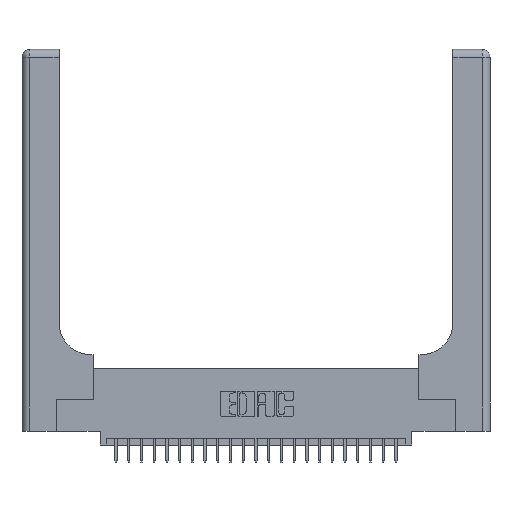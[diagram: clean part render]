
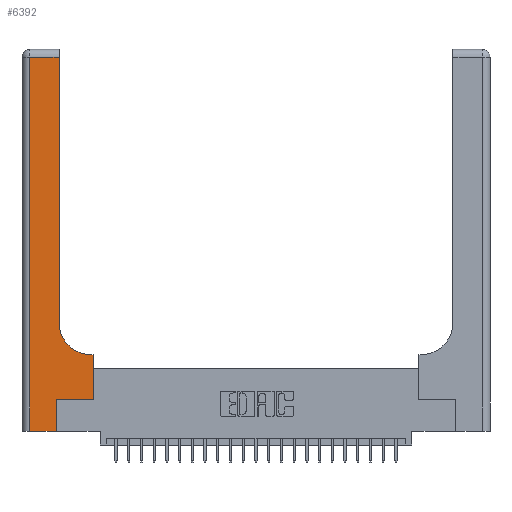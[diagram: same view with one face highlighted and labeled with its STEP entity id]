
A CAD part, top view. The second image highlights one B-rep face of the part: STEP entity #6392.
In plain terms, the highlighted planar face has unit normal (0, 0, 1).
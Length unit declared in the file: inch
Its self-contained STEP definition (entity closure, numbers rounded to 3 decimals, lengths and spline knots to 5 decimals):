
#55 = CARTESIAN_POINT ( 'NONE',  ( 0.5585, 0.25, 0.37 ) ) ;
#533 = VERTEX_POINT ( 'NONE', #17610 ) ;
#678 = CARTESIAN_POINT ( 'NONE',  ( 0.5585, 0.25, 0.37 ) ) ;
#694 = ORIENTED_EDGE ( 'NONE', *, *, #7546, .T. ) ;
#729 = LINE ( 'NONE', #22883, #1784 ) ;
#763 = DIRECTION ( 'NONE',  ( 1., 0., 0. ) ) ;
#1290 = CARTESIAN_POINT ( 'NONE',  ( 0.269, 0., 0.37 ) ) ;
#1412 = CARTESIAN_POINT ( 'NONE',  ( 0.2915, 0.85, 0.37 ) ) ;
#1784 = VECTOR ( 'NONE', #10490, 39.37008 ) ;
#1801 = DIRECTION ( 'NONE',  ( -1., 0., 0. ) ) ;
#2738 = DIRECTION ( 'NONE',  ( 0., -1., 0. ) ) ;
#2755 = ORIENTED_EDGE ( 'NONE', *, *, #14504, .T. ) ;
#3566 = CARTESIAN_POINT ( 'NONE',  ( 0.5415, 0.6, 0.37 ) ) ;
#4419 = LINE ( 'NONE', #8686, #8423 ) ;
#4421 = CARTESIAN_POINT ( 'NONE',  ( 0.269, 0.25, 0.37 ) ) ;
#4665 = LINE ( 'NONE', #6652, #6170 ) ;
#5395 = ORIENTED_EDGE ( 'NONE', *, *, #18539, .T. ) ;
#6170 = VECTOR ( 'NONE', #24715, 39.37008 ) ;
#6392 = ADVANCED_FACE ( 'NONE', ( #23810 ), #13932, .F. ) ;
#6423 = LINE ( 'NONE', #4421, #9833 ) ;
#6580 = ORIENTED_EDGE ( 'NONE', *, *, #19570, .T. ) ;
#6650 = LINE ( 'NONE', #9058, #25656 ) ;
#6652 = CARTESIAN_POINT ( 'NONE',  ( 0., 2.94, 0.37 ) ) ;
#6857 = VERTEX_POINT ( 'NONE', #10459 ) ;
#6976 = DIRECTION ( 'NONE',  ( 0., 1., 0. ) ) ;
#7003 = EDGE_LOOP ( 'NONE', ( #19323, #19224, #11215, #21803, #2755, #6580, #694, #5395, #24753 ) ) ;
#7546 = EDGE_CURVE ( 'NONE', #21017, #23763, #20070, .T. ) ;
#7895 = EDGE_CURVE ( 'NONE', #8614, #24147, #11508, .T. ) ;
#7940 = VERTEX_POINT ( 'NONE', #3566 ) ;
#8087 = DIRECTION ( 'NONE',  ( 0., 1., 0. ) ) ;
#8423 = VECTOR ( 'NONE', #2738, 39.37008 ) ;
#8614 = VERTEX_POINT ( 'NONE', #1412 ) ;
#8686 = CARTESIAN_POINT ( 'NONE',  ( 0.06, 3., 0.37 ) ) ;
#8861 = CARTESIAN_POINT ( 'NONE',  ( 0.5585, 0.6, 0.37 ) ) ;
#8979 = EDGE_CURVE ( 'NONE', #24147, #12614, #4665, .T. ) ;
#9058 = CARTESIAN_POINT ( 'NONE',  ( 0., 0., 0.37 ) ) ;
#9833 = VECTOR ( 'NONE', #763, 39.37008 ) ;
#9890 = VERTEX_POINT ( 'NONE', #1290 ) ;
#9906 = CARTESIAN_POINT ( 'NONE',  ( 0.269, 0., 0.37 ) ) ;
#10459 = CARTESIAN_POINT ( 'NONE',  ( 0.269, 0.25, 0.37 ) ) ;
#10490 = DIRECTION ( 'NONE',  ( -1., 0., 0. ) ) ;
#10966 = VECTOR ( 'NONE', #6976, 39.37008 ) ;
#11215 = ORIENTED_EDGE ( 'NONE', *, *, #13754, .T. ) ;
#11508 = LINE ( 'NONE', #21375, #18819 ) ;
#11880 = LINE ( 'NONE', #9906, #10966 ) ;
#11911 = CARTESIAN_POINT ( 'NONE',  ( 0.06, 2.94, 0.37 ) ) ;
#12614 = VERTEX_POINT ( 'NONE', #11911 ) ;
#13325 = VECTOR ( 'NONE', #8087, 39.37008 ) ;
#13754 = EDGE_CURVE ( 'NONE', #12614, #533, #4419, .T. ) ;
#13932 = PLANE ( 'NONE',  #20222 ) ;
#14504 = EDGE_CURVE ( 'NONE', #9890, #6857, #11880, .T. ) ;
#15465 = CARTESIAN_POINT ( 'NONE',  ( 0.5415, 0.85, 0.37 ) ) ;
#15857 = DIRECTION ( 'NONE',  ( 0., 0., -1. ) ) ;
#17102 = DIRECTION ( 'NONE',  ( 1., 0., 0. ) ) ;
#17264 = CARTESIAN_POINT ( 'NONE',  ( 0.2915, 2.94, 0.37 ) ) ;
#17610 = CARTESIAN_POINT ( 'NONE',  ( 0.06, 0., 0.37 ) ) ;
#17702 = DIRECTION ( 'NONE',  ( 1., 0., 0. ) ) ;
#17873 = CIRCLE ( 'NONE', #22490, 0.25 ) ;
#18539 = EDGE_CURVE ( 'NONE', #23763, #7940, #729, .T. ) ;
#18819 = VECTOR ( 'NONE', #23240, 39.37008 ) ;
#19224 = ORIENTED_EDGE ( 'NONE', *, *, #8979, .T. ) ;
#19323 = ORIENTED_EDGE ( 'NONE', *, *, #7895, .T. ) ;
#19570 = EDGE_CURVE ( 'NONE', #6857, #21017, #6423, .T. ) ;
#19989 = DIRECTION ( 'NONE',  ( 0., 0., -1. ) ) ;
#20070 = LINE ( 'NONE', #55, #13325 ) ;
#20222 = AXIS2_PLACEMENT_3D ( 'NONE', #21583, #19989, #1801 ) ;
#20771 = EDGE_CURVE ( 'NONE', #7940, #8614, #17873, .T. ) ;
#21017 = VERTEX_POINT ( 'NONE', #678 ) ;
#21375 = CARTESIAN_POINT ( 'NONE',  ( 0.2915, 3., 0.37 ) ) ;
#21583 = CARTESIAN_POINT ( 'NONE',  ( 0., 3., 0.37 ) ) ;
#21803 = ORIENTED_EDGE ( 'NONE', *, *, #24566, .T. ) ;
#22490 = AXIS2_PLACEMENT_3D ( 'NONE', #15465, #15857, #17702 ) ;
#22883 = CARTESIAN_POINT ( 'NONE',  ( 0.2915, 0.6, 0.37 ) ) ;
#23240 = DIRECTION ( 'NONE',  ( 0., 1., 0. ) ) ;
#23763 = VERTEX_POINT ( 'NONE', #8861 ) ;
#23810 = FACE_OUTER_BOUND ( 'NONE', #7003, .T. ) ;
#24147 = VERTEX_POINT ( 'NONE', #17264 ) ;
#24566 = EDGE_CURVE ( 'NONE', #533, #9890, #6650, .T. ) ;
#24715 = DIRECTION ( 'NONE',  ( -1., 0., 0. ) ) ;
#24753 = ORIENTED_EDGE ( 'NONE', *, *, #20771, .T. ) ;
#25656 = VECTOR ( 'NONE', #17102, 39.37008 ) ;
